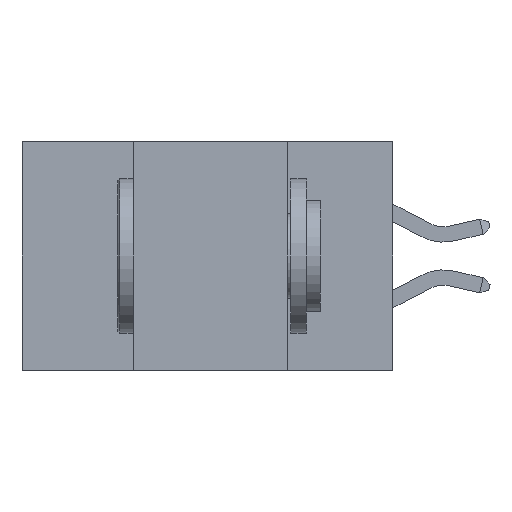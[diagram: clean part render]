
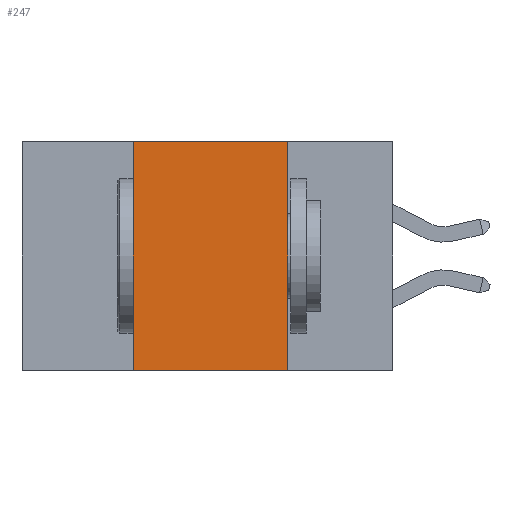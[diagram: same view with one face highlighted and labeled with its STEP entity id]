
A CAD part, left-side view. The second image highlights one B-rep face of the part: STEP entity #247.
In plain terms, the highlighted planar face has unit normal (-1, 0, 0).
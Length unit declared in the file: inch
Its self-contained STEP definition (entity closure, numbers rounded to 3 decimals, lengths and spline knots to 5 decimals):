
#220 = CARTESIAN_POINT ( 'NONE',  ( 0., 0.42, 0. ) ) ;
#247 = ADVANCED_FACE ( 'NONE', ( #13832 ), #11217, .F. ) ;
#387 = DIRECTION ( 'NONE',  ( 0., 0., -1. ) ) ;
#541 = VECTOR ( 'NONE', #1019, 39.37008 ) ;
#1019 = DIRECTION ( 'NONE',  ( 0., -1., 0. ) ) ;
#1709 = CARTESIAN_POINT ( 'NONE',  ( 0., 0.17, 0. ) ) ;
#1716 = VECTOR ( 'NONE', #6855, 39.37008 ) ;
#3193 = DIRECTION ( 'NONE',  ( 1., 0., 0. ) ) ;
#3331 = CARTESIAN_POINT ( 'NONE',  ( 0., 0.42, -0.37 ) ) ;
#3953 = ORIENTED_EDGE ( 'NONE', *, *, #12397, .T. ) ;
#4486 = CARTESIAN_POINT ( 'NONE',  ( 0., 0.6, -0.37 ) ) ;
#5648 = EDGE_CURVE ( 'NONE', #6505, #8898, #12283, .T. ) ;
#6001 = VERTEX_POINT ( 'NONE', #3331 ) ;
#6505 = VERTEX_POINT ( 'NONE', #1709 ) ;
#6832 = EDGE_CURVE ( 'NONE', #14502, #6505, #15163, .T. ) ;
#6855 = DIRECTION ( 'NONE',  ( 0., 0., -1. ) ) ;
#7170 = ORIENTED_EDGE ( 'NONE', *, *, #12954, .F. ) ;
#7271 = CARTESIAN_POINT ( 'NONE',  ( 0., 0.42, 0. ) ) ;
#7477 = AXIS2_PLACEMENT_3D ( 'NONE', #16348, #3193, #387 ) ;
#8332 = CARTESIAN_POINT ( 'NONE',  ( 0., 0.17, -0.37 ) ) ;
#8898 = VERTEX_POINT ( 'NONE', #8332 ) ;
#9899 = LINE ( 'NONE', #7271, #13064 ) ;
#9962 = ORIENTED_EDGE ( 'NONE', *, *, #5648, .F. ) ;
#10028 = DIRECTION ( 'NONE',  ( 0., 0., 1. ) ) ;
#11205 = LINE ( 'NONE', #4486, #14336 ) ;
#11217 = PLANE ( 'NONE',  #7477 ) ;
#11303 = DIRECTION ( 'NONE',  ( 0., -1., 0. ) ) ;
#12283 = LINE ( 'NONE', #12288, #1716 ) ;
#12288 = CARTESIAN_POINT ( 'NONE',  ( 0., 0.17, 0. ) ) ;
#12397 = EDGE_CURVE ( 'NONE', #6001, #8898, #11205, .T. ) ;
#12954 = EDGE_CURVE ( 'NONE', #6001, #14502, #9899, .T. ) ;
#13064 = VECTOR ( 'NONE', #10028, 39.37008 ) ;
#13832 = FACE_OUTER_BOUND ( 'NONE', #14647, .T. ) ;
#13968 = ORIENTED_EDGE ( 'NONE', *, *, #6832, .F. ) ;
#14336 = VECTOR ( 'NONE', #11303, 39.37008 ) ;
#14502 = VERTEX_POINT ( 'NONE', #220 ) ;
#14647 = EDGE_LOOP ( 'NONE', ( #9962, #13968, #7170, #3953 ) ) ;
#15163 = LINE ( 'NONE', #17371, #541 ) ;
#16348 = CARTESIAN_POINT ( 'NONE',  ( 0., 0.6, 0. ) ) ;
#17371 = CARTESIAN_POINT ( 'NONE',  ( 0., 0.6, 0. ) ) ;
